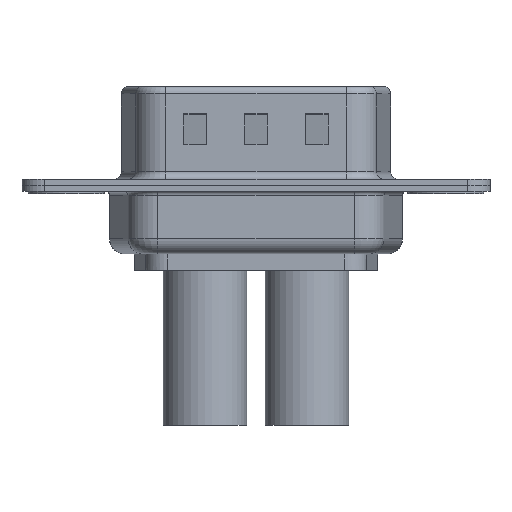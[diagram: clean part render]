
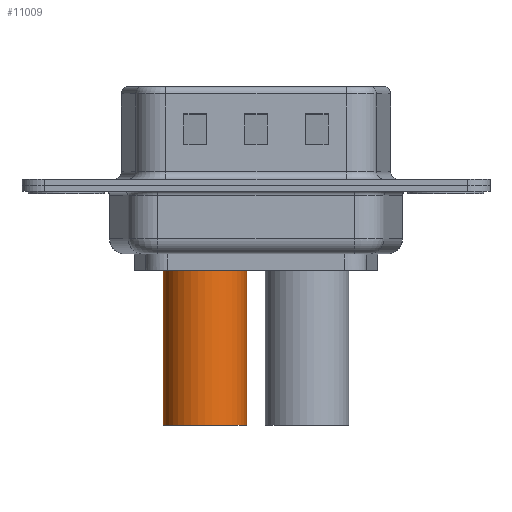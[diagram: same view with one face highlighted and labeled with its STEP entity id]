
A CAD part, front view. The second image highlights one B-rep face of the part: STEP entity #11009.
In plain terms, the highlighted cylindrical face has radius 2.75 mm (diameter 5.5 mm), a partial arc.
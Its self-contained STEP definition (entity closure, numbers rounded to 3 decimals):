
#619 = DIRECTION ( 'NONE',  ( 1., 0., 0. ) ) ;
#934 = VERTEX_POINT ( 'NONE', #11103 ) ;
#2293 = DIRECTION ( 'NONE',  ( 0., 0., 1. ) ) ;
#2521 = CIRCLE ( 'NONE', #2569, 2.75 ) ;
#2552 = CYLINDRICAL_SURFACE ( 'NONE', #5819, 2.75 ) ;
#2569 = AXIS2_PLACEMENT_3D ( 'NONE', #4564, #6729, #8754 ) ;
#3060 = VERTEX_POINT ( 'NONE', #3829 ) ;
#3229 = FACE_OUTER_BOUND ( 'NONE', #8234, .T. ) ;
#3387 = CARTESIAN_POINT ( 'NONE',  ( -2.75, 0., 4.234 ) ) ;
#3829 = CARTESIAN_POINT ( 'NONE',  ( -2.75, 0., 1.5 ) ) ;
#4161 = CIRCLE ( 'NONE', #10137, 2.75 ) ;
#4417 = ORIENTED_EDGE ( 'NONE', *, *, #6604, .F. ) ;
#4564 = CARTESIAN_POINT ( 'NONE',  ( 0., 0., 1.5 ) ) ;
#4692 = LINE ( 'NONE', #7348, #9432 ) ;
#4792 = LINE ( 'NONE', #6387, #11937 ) ;
#5241 = DIRECTION ( 'NONE',  ( 1., 0., 0. ) ) ;
#5270 = EDGE_CURVE ( 'NONE', #3060, #6370, #2521, .T. ) ;
#5371 = DIRECTION ( 'NONE',  ( 0., 0., -1. ) ) ;
#5609 = ORIENTED_EDGE ( 'NONE', *, *, #5270, .F. ) ;
#5722 = CARTESIAN_POINT ( 'NONE',  ( 2.75, 0., 4.234 ) ) ;
#5771 = CARTESIAN_POINT ( 'NONE',  ( -2.75, 0., -8.7 ) ) ;
#5819 = AXIS2_PLACEMENT_3D ( 'NONE', #6603, #6817, #619 ) ;
#5902 = VERTEX_POINT ( 'NONE', #7372 ) ;
#6057 = CARTESIAN_POINT ( 'NONE',  ( 0., 0., -8.7 ) ) ;
#6071 = EDGE_CURVE ( 'NONE', #934, #6370, #9443, .T. ) ;
#6370 = VERTEX_POINT ( 'NONE', #9485 ) ;
#6387 = CARTESIAN_POINT ( 'NONE',  ( -2.75, 0., -8.7 ) ) ;
#6603 = CARTESIAN_POINT ( 'NONE',  ( 0., 0., 4.234 ) ) ;
#6604 = EDGE_CURVE ( 'NONE', #934, #9786, #4692, .T. ) ;
#6729 = DIRECTION ( 'NONE',  ( 0., 0., 1. ) ) ;
#6817 = DIRECTION ( 'NONE',  ( 0., 0., 1. ) ) ;
#7251 = EDGE_CURVE ( 'NONE', #11505, #9786, #4161, .T. ) ;
#7348 = CARTESIAN_POINT ( 'NONE',  ( 2.75, 0., -8.7 ) ) ;
#7372 = CARTESIAN_POINT ( 'NONE',  ( -2.75, 0., -7.764 ) ) ;
#7486 = ORIENTED_EDGE ( 'NONE', *, *, #6071, .T. ) ;
#8133 = DIRECTION ( 'NONE',  ( 0., 0., 1. ) ) ;
#8234 = EDGE_LOOP ( 'NONE', ( #9326, #11306, #11741, #4417, #7486, #5609 ) ) ;
#8605 = EDGE_CURVE ( 'NONE', #5902, #3060, #10388, .T. ) ;
#8754 = DIRECTION ( 'NONE',  ( 1., 0., 0. ) ) ;
#9084 = EDGE_CURVE ( 'NONE', #5902, #11505, #4792, .T. ) ;
#9326 = ORIENTED_EDGE ( 'NONE', *, *, #8605, .F. ) ;
#9379 = DIRECTION ( 'NONE',  ( 0., 0., -1. ) ) ;
#9432 = VECTOR ( 'NONE', #9379, 1000. ) ;
#9443 = LINE ( 'NONE', #5722, #12180 ) ;
#9474 = DIRECTION ( 'NONE',  ( 0., 0., 1. ) ) ;
#9485 = CARTESIAN_POINT ( 'NONE',  ( 2.75, 0., 1.5 ) ) ;
#9786 = VERTEX_POINT ( 'NONE', #12369 ) ;
#9809 = VECTOR ( 'NONE', #2293, 1000. ) ;
#10137 = AXIS2_PLACEMENT_3D ( 'NONE', #6057, #8133, #5241 ) ;
#10388 = LINE ( 'NONE', #3387, #9809 ) ;
#11009 = ADVANCED_FACE ( 'NONE', ( #3229 ), #2552, .T. ) ;
#11103 = CARTESIAN_POINT ( 'NONE',  ( 2.75, 0., -7.764 ) ) ;
#11306 = ORIENTED_EDGE ( 'NONE', *, *, #9084, .T. ) ;
#11505 = VERTEX_POINT ( 'NONE', #5771 ) ;
#11741 = ORIENTED_EDGE ( 'NONE', *, *, #7251, .T. ) ;
#11937 = VECTOR ( 'NONE', #5371, 1000. ) ;
#12180 = VECTOR ( 'NONE', #9474, 1000. ) ;
#12369 = CARTESIAN_POINT ( 'NONE',  ( 2.75, 0., -8.7 ) ) ;
